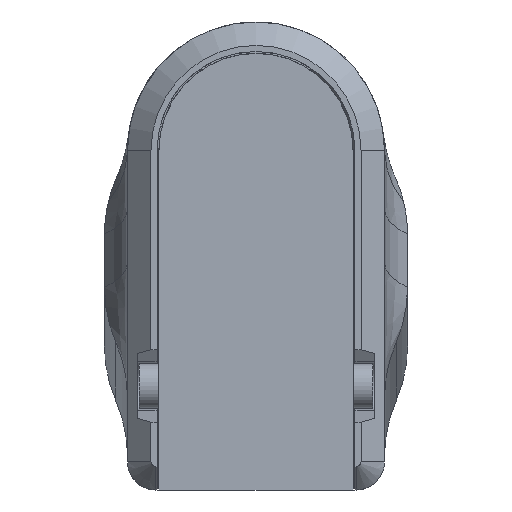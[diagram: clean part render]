
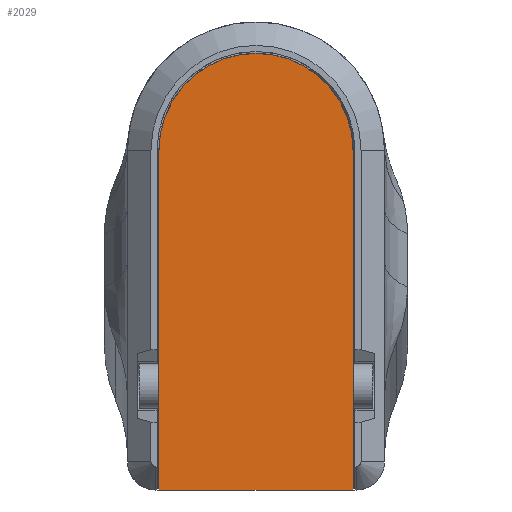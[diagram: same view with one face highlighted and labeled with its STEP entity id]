
A CAD part, front view. The second image highlights one B-rep face of the part: STEP entity #2029.
In plain terms, the highlighted planar face has unit normal (0, -1, 0).
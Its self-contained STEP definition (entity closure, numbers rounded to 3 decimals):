
#131=PLANE('',#2189);
#195=FACE_OUTER_BOUND('',#320,.T.);
#320=EDGE_LOOP('',(#1462,#1463,#1464,#1465));
#459=LINE('',#3009,#639);
#464=LINE('',#3020,#644);
#465=LINE('',#3022,#645);
#639=VECTOR('',#2438,10.);
#644=VECTOR('',#2451,10.);
#645=VECTOR('',#2454,10.);
#798=CIRCLE('',#2185,10.35);
#899=VERTEX_POINT('',#3006);
#900=VERTEX_POINT('',#3008);
#901=VERTEX_POINT('',#3012);
#902=VERTEX_POINT('',#3018);
#1103=EDGE_CURVE('',#900,#899,#459,.T.);
#1106=EDGE_CURVE('',#899,#901,#798,.T.);
#1109=EDGE_CURVE('',#900,#902,#464,.T.);
#1110=EDGE_CURVE('',#902,#901,#465,.T.);
#1462=ORIENTED_EDGE('',*,*,#1106,.T.);
#1463=ORIENTED_EDGE('',*,*,#1110,.F.);
#1464=ORIENTED_EDGE('',*,*,#1109,.F.);
#1465=ORIENTED_EDGE('',*,*,#1103,.T.);
#2029=ADVANCED_FACE('',(#195),#131,.F.);
#2185=AXIS2_PLACEMENT_3D('',#3014,#2443,#2444);
#2189=AXIS2_PLACEMENT_3D('',#3023,#2455,#2456);
#2438=DIRECTION('',(0.,0.,1.));
#2443=DIRECTION('center_axis',(0.,-1.,0.));
#2444=DIRECTION('ref_axis',(-1.,0.,0.));
#2451=DIRECTION('',(-1.,0.,0.));
#2454=DIRECTION('',(0.,0.,1.));
#2455=DIRECTION('center_axis',(0.,1.,0.));
#2456=DIRECTION('ref_axis',(1.,0.,0.));
#3006=CARTESIAN_POINT('',(10.35,0.,36.2));
#3008=CARTESIAN_POINT('',(10.35,0.,0.));
#3009=CARTESIAN_POINT('',(10.35,0.,0.));
#3012=CARTESIAN_POINT('',(-10.35,0.,36.2));
#3014=CARTESIAN_POINT('Origin',(0.,0.,36.2));
#3018=CARTESIAN_POINT('',(-10.35,0.,0.));
#3020=CARTESIAN_POINT('',(10.35,0.,0.));
#3022=CARTESIAN_POINT('',(-10.35,0.,0.));
#3023=CARTESIAN_POINT('Origin',(0.,0.,23.275));
